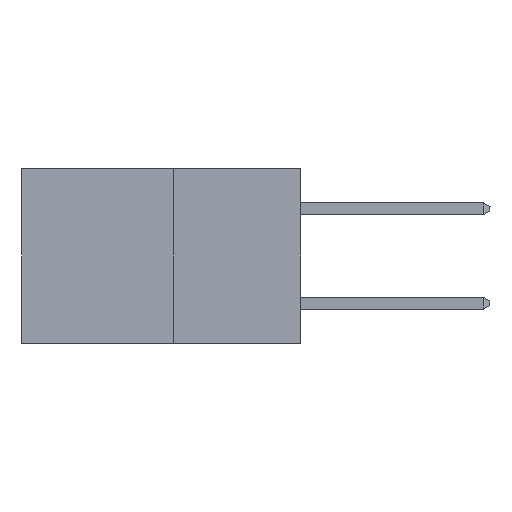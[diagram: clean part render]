
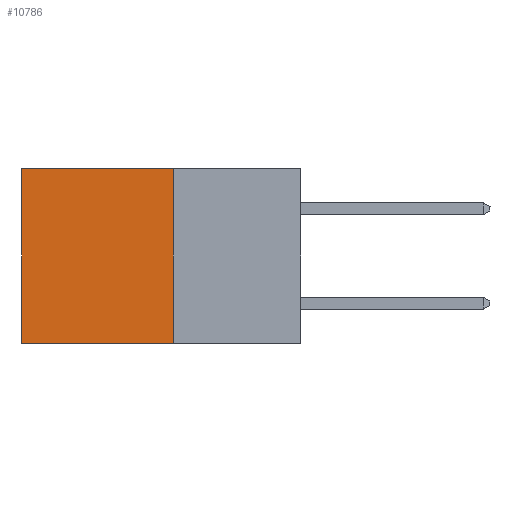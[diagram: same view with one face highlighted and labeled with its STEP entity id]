
A CAD part, left-side view. The second image highlights one B-rep face of the part: STEP entity #10786.
In plain terms, the highlighted planar face has unit normal (-1, 0, 0).
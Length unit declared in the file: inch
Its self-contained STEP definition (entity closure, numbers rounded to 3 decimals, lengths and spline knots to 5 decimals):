
#679 = CARTESIAN_POINT ( 'NONE',  ( 0.277, 0.27, 0. ) ) ;
#695 = DIRECTION ( 'NONE',  ( 0., 1., 0. ) ) ;
#1397 = CARTESIAN_POINT ( 'NONE',  ( 0.277, 0.59, -0.37 ) ) ;
#1708 = CARTESIAN_POINT ( 'NONE',  ( 0.277, 0.59, -0.37 ) ) ;
#1769 = LINE ( 'NONE', #679, #7481 ) ;
#2001 = CARTESIAN_POINT ( 'NONE',  ( 0.277, 0.27, 0. ) ) ;
#2004 = DIRECTION ( 'NONE',  ( 0., 0., -1. ) ) ;
#2048 = PLANE ( 'NONE',  #10970 ) ;
#2497 = EDGE_CURVE ( 'NONE', #10777, #3013, #7128, .T. ) ;
#3013 = VERTEX_POINT ( 'NONE', #3902 ) ;
#3145 = DIRECTION ( 'NONE',  ( 0., 1., 0. ) ) ;
#3329 = CARTESIAN_POINT ( 'NONE',  ( 0.277, 0.27, -0.37 ) ) ;
#3902 = CARTESIAN_POINT ( 'NONE',  ( 0.277, 0.27, -0.37 ) ) ;
#4487 = CARTESIAN_POINT ( 'NONE',  ( 0.277, 0.27, -0.37 ) ) ;
#4590 = VECTOR ( 'NONE', #3145, 39.37008 ) ;
#5152 = ORIENTED_EDGE ( 'NONE', *, *, #2497, .F. ) ;
#5432 = CARTESIAN_POINT ( 'NONE',  ( 0.277, 0.27, -0.37 ) ) ;
#5534 = DIRECTION ( 'NONE',  ( 0., 0., -1. ) ) ;
#5720 = DIRECTION ( 'NONE',  ( 0., 0., -1. ) ) ;
#6724 = VECTOR ( 'NONE', #5534, 39.37008 ) ;
#7128 = LINE ( 'NONE', #5432, #6724 ) ;
#7481 = VECTOR ( 'NONE', #695, 39.37008 ) ;
#7676 = EDGE_CURVE ( 'NONE', #11399, #12815, #11579, .T. ) ;
#8826 = EDGE_CURVE ( 'NONE', #3013, #12815, #10632, .T. ) ;
#9036 = EDGE_CURVE ( 'NONE', #10777, #11399, #1769, .T. ) ;
#9837 = EDGE_LOOP ( 'NONE', ( #15091, #11144, #5152, #15519 ) ) ;
#10632 = LINE ( 'NONE', #3329, #4590 ) ;
#10777 = VERTEX_POINT ( 'NONE', #2001 ) ;
#10786 = ADVANCED_FACE ( 'NONE', ( #12713 ), #2048, .F. ) ;
#10970 = AXIS2_PLACEMENT_3D ( 'NONE', #4487, #12907, #5720 ) ;
#11144 = ORIENTED_EDGE ( 'NONE', *, *, #8826, .F. ) ;
#11399 = VERTEX_POINT ( 'NONE', #11556 ) ;
#11556 = CARTESIAN_POINT ( 'NONE',  ( 0.277, 0.59, 0. ) ) ;
#11579 = LINE ( 'NONE', #1397, #15175 ) ;
#12713 = FACE_OUTER_BOUND ( 'NONE', #9837, .T. ) ;
#12815 = VERTEX_POINT ( 'NONE', #1708 ) ;
#12907 = DIRECTION ( 'NONE',  ( 1., 0., 0. ) ) ;
#15091 = ORIENTED_EDGE ( 'NONE', *, *, #7676, .T. ) ;
#15175 = VECTOR ( 'NONE', #2004, 39.37008 ) ;
#15519 = ORIENTED_EDGE ( 'NONE', *, *, #9036, .T. ) ;
